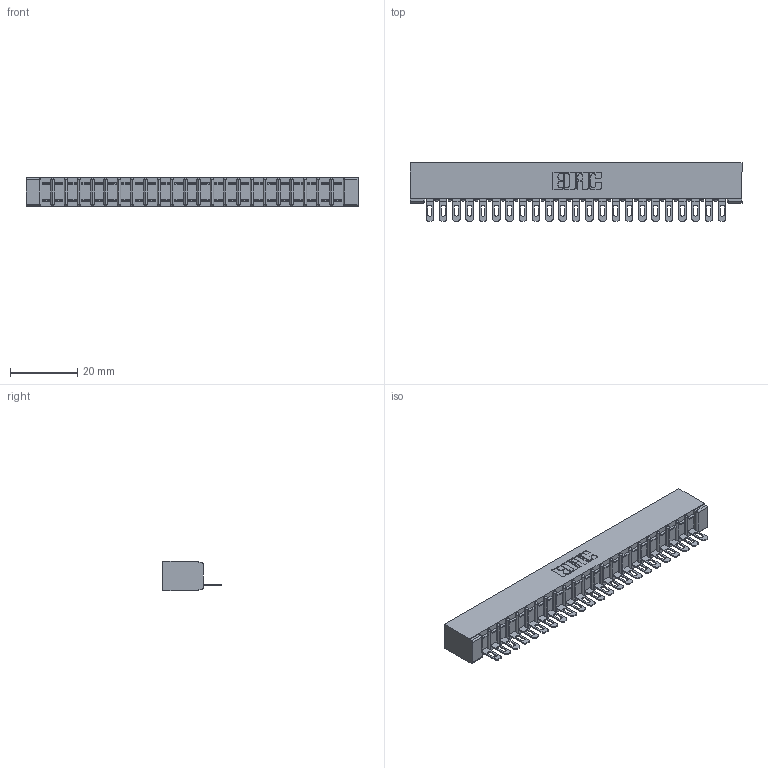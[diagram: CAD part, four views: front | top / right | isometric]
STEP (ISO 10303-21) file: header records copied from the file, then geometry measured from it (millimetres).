
FILE_DESCRIPTION (( 'STEP AP203' ), '1' );
FILE_NAME ('307-023-501-101.STEP', '2019-09-05T00:19:37', ( '' ), ( '' ), 'SwSTEP 2.0', 'SolidWorks 2016', '' );
FILE_SCHEMA (( 'CONFIG_CONTROL_DESIGN' ));
Length unit declared in the file: inch
Products named in the file (3): 307-023-501-101; 307 Part_No Mounting Lugs; 307-290-002_501
Assembly tree (24 placements, depth 2):
  307-023-501-101
    307 Part_No Mounting Lugs
    307-290-002_501  x23
Bounding box: 99.01 x 17.42 x 8.71 mm (x, y, z)
Volume: 6799.3 mm3; surface area: 13084.3 mm2
Topology: 24 solids, 24 shells, 1882 faces, 5773 edges, 3782 vertices
Faces by surface type: plane 1078, cylinder 756, sphere 48
Entity records: 22576 total; most frequent: CARTESIAN_POINT 3804, ORIENTED_EDGE 3794, DIRECTION 3707, EDGE_CURVE 1897, LINE 1441, VECTOR 1441, VERTEX_POINT 1230, AXIS2_PLACEMENT_3D 1133
